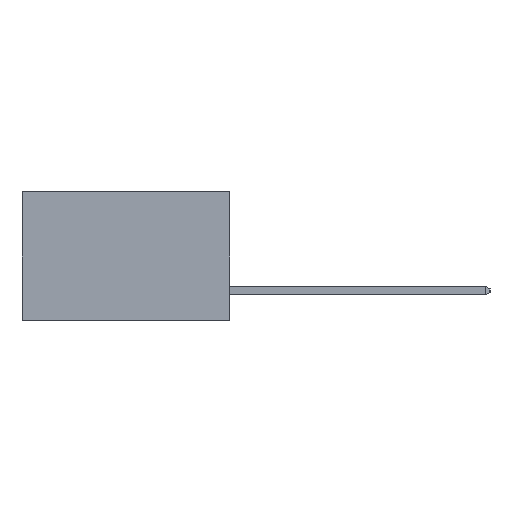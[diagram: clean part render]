
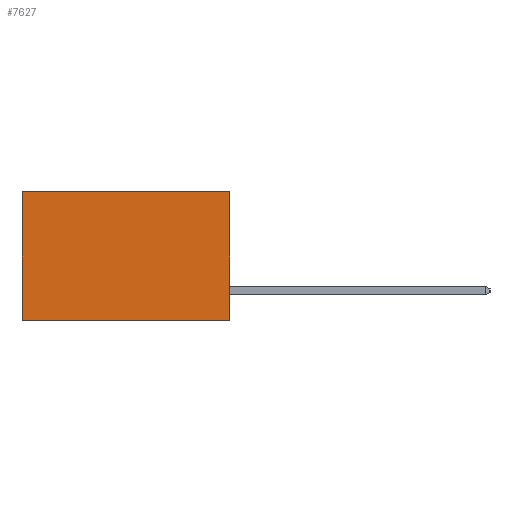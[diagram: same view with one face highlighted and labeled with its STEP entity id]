
A CAD part, left-side view. The second image highlights one B-rep face of the part: STEP entity #7627.
In plain terms, the highlighted planar face has unit normal (-1, 0, 0).
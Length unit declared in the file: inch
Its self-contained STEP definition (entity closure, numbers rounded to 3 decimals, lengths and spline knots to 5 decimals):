
#293 = VERTEX_POINT ( 'NONE', #10425 ) ;
#1067 = DIRECTION ( 'NONE',  ( 0., 0., -1. ) ) ;
#1684 = AXIS2_PLACEMENT_3D ( 'NONE', #3426, #6984, #14661 ) ;
#2391 = CARTESIAN_POINT ( 'NONE',  ( 0.2615, 0., 0. ) ) ;
#2430 = ORIENTED_EDGE ( 'NONE', *, *, #13155, .T. ) ;
#2543 = CARTESIAN_POINT ( 'NONE',  ( 0.2615, 0., -0.37 ) ) ;
#2648 = DIRECTION ( 'NONE',  ( 0., 0., -1. ) ) ;
#2655 = CARTESIAN_POINT ( 'NONE',  ( 0.2615, 0., -0.37 ) ) ;
#2687 = EDGE_CURVE ( 'NONE', #12729, #7070, #7676, .T. ) ;
#3426 = CARTESIAN_POINT ( 'NONE',  ( 0.2615, 0., -0.37 ) ) ;
#3747 = DIRECTION ( 'NONE',  ( 0., 1., 0. ) ) ;
#4118 = ORIENTED_EDGE ( 'NONE', *, *, #11550, .F. ) ;
#4981 = VECTOR ( 'NONE', #14774, 39.37008 ) ;
#5838 = PLANE ( 'NONE',  #1684 ) ;
#5921 = ORIENTED_EDGE ( 'NONE', *, *, #2687, .F. ) ;
#6171 = VECTOR ( 'NONE', #3747, 39.37008 ) ;
#6984 = DIRECTION ( 'NONE',  ( 1., 0., 0. ) ) ;
#7070 = VERTEX_POINT ( 'NONE', #14123 ) ;
#7627 = ADVANCED_FACE ( 'NONE', ( #13071 ), #5838, .F. ) ;
#7676 = LINE ( 'NONE', #2655, #8045 ) ;
#8045 = VECTOR ( 'NONE', #2648, 39.37008 ) ;
#8189 = EDGE_CURVE ( 'NONE', #12729, #13248, #11051, .T. ) ;
#8627 = VECTOR ( 'NONE', #1067, 39.37008 ) ;
#9191 = ORIENTED_EDGE ( 'NONE', *, *, #8189, .T. ) ;
#9348 = CARTESIAN_POINT ( 'NONE',  ( 0.2615, 0.6, -0.37 ) ) ;
#10425 = CARTESIAN_POINT ( 'NONE',  ( 0.2615, 0.6, -0.37 ) ) ;
#11051 = LINE ( 'NONE', #2391, #4981 ) ;
#11417 = EDGE_LOOP ( 'NONE', ( #2430, #4118, #5921, #9191 ) ) ;
#11438 = LINE ( 'NONE', #2543, #6171 ) ;
#11550 = EDGE_CURVE ( 'NONE', #7070, #293, #11438, .T. ) ;
#11557 = LINE ( 'NONE', #9348, #8627 ) ;
#12729 = VERTEX_POINT ( 'NONE', #14105 ) ;
#13071 = FACE_OUTER_BOUND ( 'NONE', #11417, .T. ) ;
#13155 = EDGE_CURVE ( 'NONE', #13248, #293, #11557, .T. ) ;
#13248 = VERTEX_POINT ( 'NONE', #13812 ) ;
#13812 = CARTESIAN_POINT ( 'NONE',  ( 0.2615, 0.6, 0. ) ) ;
#14105 = CARTESIAN_POINT ( 'NONE',  ( 0.2615, 0., 0. ) ) ;
#14123 = CARTESIAN_POINT ( 'NONE',  ( 0.2615, 0., -0.37 ) ) ;
#14661 = DIRECTION ( 'NONE',  ( 0., 0., -1. ) ) ;
#14774 = DIRECTION ( 'NONE',  ( 0., 1., 0. ) ) ;
